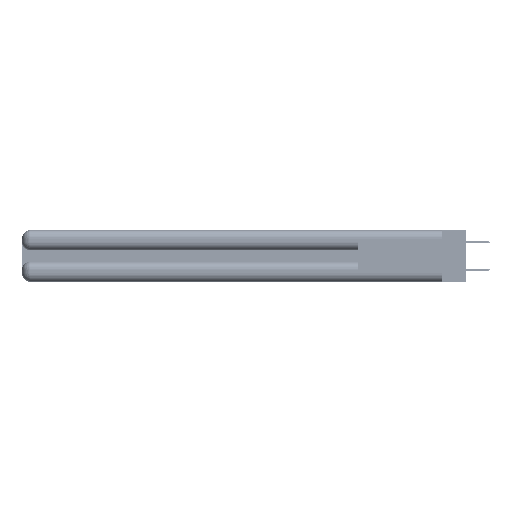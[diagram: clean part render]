
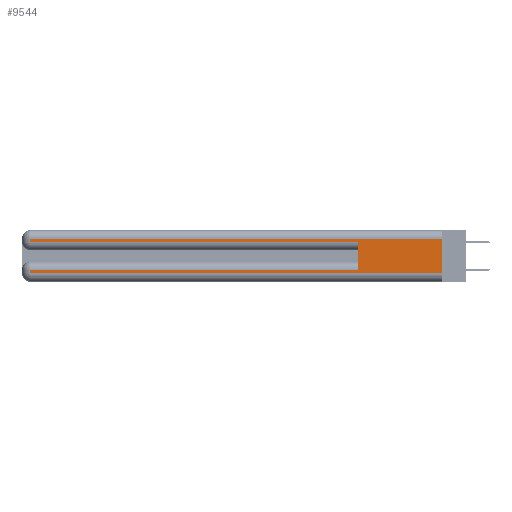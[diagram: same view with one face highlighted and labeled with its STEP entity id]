
A CAD part, left-side view. The second image highlights one B-rep face of the part: STEP entity #9544.
In plain terms, the highlighted planar face has unit normal (-1, 0, 0).
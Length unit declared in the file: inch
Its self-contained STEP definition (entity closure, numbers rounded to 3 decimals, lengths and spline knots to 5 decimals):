
#200 = VECTOR ( 'NONE', #17389, 39.37008 ) ;
#330 = EDGE_CURVE ( 'NONE', #30689, #21492, #6877, .T. ) ;
#457 = EDGE_CURVE ( 'NONE', #2070, #13446, #29171, .T. ) ;
#1631 = ORIENTED_EDGE ( 'NONE', *, *, #16507, .T. ) ;
#1729 = LINE ( 'NONE', #17584, #21411 ) ;
#1808 = CARTESIAN_POINT ( 'NONE',  ( 0., 0.6, 0.285 ) ) ;
#2070 = VERTEX_POINT ( 'NONE', #11758 ) ;
#3956 = CARTESIAN_POINT ( 'NONE',  ( 0., 2.94, 0.085 ) ) ;
#4909 = CARTESIAN_POINT ( 'NONE',  ( 0., 0., 0.37 ) ) ;
#6115 = CARTESIAN_POINT ( 'NONE',  ( 0., 0.6, 0.085 ) ) ;
#6877 = LINE ( 'NONE', #32261, #44943 ) ;
#8556 = CARTESIAN_POINT ( 'NONE',  ( 0., 0., 0.285 ) ) ;
#9544 = ADVANCED_FACE ( 'NONE', ( #23935 ), #36401, .F. ) ;
#9857 = DIRECTION ( 'NONE',  ( 0., 0., -1. ) ) ;
#11758 = CARTESIAN_POINT ( 'NONE',  ( 0., 2.94, 0.06 ) ) ;
#11982 = LINE ( 'NONE', #41562, #13215 ) ;
#12823 = DIRECTION ( 'NONE',  ( 1., 0., 0. ) ) ;
#13215 = VECTOR ( 'NONE', #14067, 39.37008 ) ;
#13391 = EDGE_CURVE ( 'NONE', #39399, #43379, #24849, .T. ) ;
#13446 = VERTEX_POINT ( 'NONE', #43339 ) ;
#14067 = DIRECTION ( 'NONE',  ( 0., 0., -1. ) ) ;
#14475 = CARTESIAN_POINT ( 'NONE',  ( 0., 2.94, 0.31 ) ) ;
#15526 = EDGE_CURVE ( 'NONE', #21492, #46138, #25251, .T. ) ;
#16311 = LINE ( 'NONE', #34460, #37223 ) ;
#16507 = EDGE_CURVE ( 'NONE', #43379, #2070, #1729, .T. ) ;
#17048 = LINE ( 'NONE', #29676, #36751 ) ;
#17389 = DIRECTION ( 'NONE',  ( 0., -1., 0. ) ) ;
#17584 = CARTESIAN_POINT ( 'NONE',  ( 0., 2.94, 0.37 ) ) ;
#18252 = EDGE_CURVE ( 'NONE', #35737, #13446, #11982, .T. ) ;
#18609 = DIRECTION ( 'NONE',  ( 0., 1., 0. ) ) ;
#19824 = ORIENTED_EDGE ( 'NONE', *, *, #26981, .T. ) ;
#21411 = VECTOR ( 'NONE', #9857, 39.37008 ) ;
#21492 = VERTEX_POINT ( 'NONE', #40632 ) ;
#23935 = FACE_OUTER_BOUND ( 'NONE', #49662, .T. ) ;
#24849 = LINE ( 'NONE', #31258, #44411 ) ;
#25251 = LINE ( 'NONE', #8556, #45986 ) ;
#26981 = EDGE_CURVE ( 'NONE', #35737, #30689, #16311, .T. ) ;
#27379 = ORIENTED_EDGE ( 'NONE', *, *, #18252, .F. ) ;
#29171 = LINE ( 'NONE', #37178, #200 ) ;
#29676 = CARTESIAN_POINT ( 'NONE',  ( 0., 0.6, 0.145 ) ) ;
#30689 = VERTEX_POINT ( 'NONE', #14475 ) ;
#31258 = CARTESIAN_POINT ( 'NONE',  ( 0., 0., 0.085 ) ) ;
#31418 = DIRECTION ( 'NONE',  ( 0., 1., 0. ) ) ;
#32261 = CARTESIAN_POINT ( 'NONE',  ( 0., 2.94, 0.37 ) ) ;
#33598 = DIRECTION ( 'NONE',  ( 0., 0., 1. ) ) ;
#34460 = CARTESIAN_POINT ( 'NONE',  ( 0., 0., 0.31 ) ) ;
#35737 = VERTEX_POINT ( 'NONE', #43621 ) ;
#36093 = DIRECTION ( 'NONE',  ( 0., -1., 0. ) ) ;
#36177 = DIRECTION ( 'NONE',  ( 0., 0., -1. ) ) ;
#36401 = PLANE ( 'NONE',  #43523 ) ;
#36751 = VECTOR ( 'NONE', #33598, 39.37008 ) ;
#37178 = CARTESIAN_POINT ( 'NONE',  ( 0., 0., 0.06 ) ) ;
#37223 = VECTOR ( 'NONE', #18609, 39.37008 ) ;
#37516 = ORIENTED_EDGE ( 'NONE', *, *, #330, .T. ) ;
#38543 = ORIENTED_EDGE ( 'NONE', *, *, #15526, .T. ) ;
#39399 = VERTEX_POINT ( 'NONE', #6115 ) ;
#39956 = EDGE_CURVE ( 'NONE', #39399, #46138, #17048, .T. ) ;
#40293 = DIRECTION ( 'NONE',  ( 0., 0., -1. ) ) ;
#40632 = CARTESIAN_POINT ( 'NONE',  ( 0., 2.94, 0.285 ) ) ;
#41562 = CARTESIAN_POINT ( 'NONE',  ( 0., 0., 0.37 ) ) ;
#41869 = ORIENTED_EDGE ( 'NONE', *, *, #39956, .F. ) ;
#43339 = CARTESIAN_POINT ( 'NONE',  ( 0., 0., 0.06 ) ) ;
#43379 = VERTEX_POINT ( 'NONE', #3956 ) ;
#43523 = AXIS2_PLACEMENT_3D ( 'NONE', #4909, #12823, #40293 ) ;
#43621 = CARTESIAN_POINT ( 'NONE',  ( 0., 0., 0.31 ) ) ;
#44411 = VECTOR ( 'NONE', #31418, 39.37008 ) ;
#44760 = ORIENTED_EDGE ( 'NONE', *, *, #457, .T. ) ;
#44943 = VECTOR ( 'NONE', #36177, 39.37008 ) ;
#45467 = ORIENTED_EDGE ( 'NONE', *, *, #13391, .T. ) ;
#45986 = VECTOR ( 'NONE', #36093, 39.37008 ) ;
#46138 = VERTEX_POINT ( 'NONE', #1808 ) ;
#49662 = EDGE_LOOP ( 'NONE', ( #27379, #19824, #37516, #38543, #41869, #45467, #1631, #44760 ) ) ;
